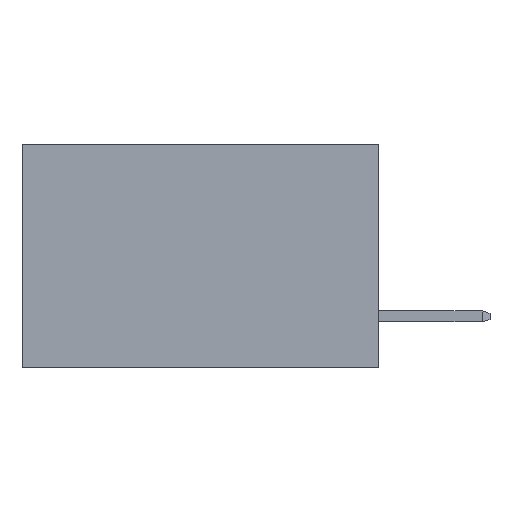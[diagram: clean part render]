
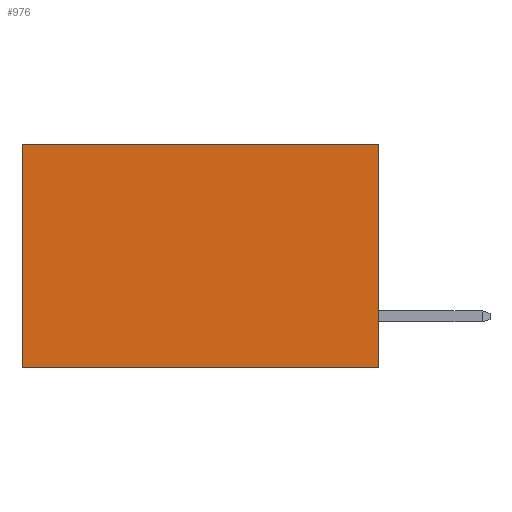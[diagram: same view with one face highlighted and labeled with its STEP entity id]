
A CAD part, left-side view. The second image highlights one B-rep face of the part: STEP entity #976.
In plain terms, the highlighted planar face has unit normal (-1, 0, 0).
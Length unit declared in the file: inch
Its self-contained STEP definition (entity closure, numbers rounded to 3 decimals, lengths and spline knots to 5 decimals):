
#169 = CARTESIAN_POINT ( 'NONE',  ( 0.277, 0., -0.37 ) ) ;
#976 = ADVANCED_FACE ( 'NONE', ( #1523 ), #10829, .F. ) ;
#1224 = DIRECTION ( 'NONE',  ( 0., 1., 0. ) ) ;
#1523 = FACE_OUTER_BOUND ( 'NONE', #5563, .T. ) ;
#1604 = EDGE_CURVE ( 'NONE', #8723, #1675, #9180, .T. ) ;
#1675 = VERTEX_POINT ( 'NONE', #10367 ) ;
#1906 = ORIENTED_EDGE ( 'NONE', *, *, #6919, .F. ) ;
#2808 = VECTOR ( 'NONE', #1224, 39.37008 ) ;
#2923 = EDGE_CURVE ( 'NONE', #1675, #7346, #4259, .T. ) ;
#3190 = CARTESIAN_POINT ( 'NONE',  ( 0.277, 0., 0. ) ) ;
#3775 = DIRECTION ( 'NONE',  ( 0., 0., -1. ) ) ;
#3964 = ORIENTED_EDGE ( 'NONE', *, *, #2923, .T. ) ;
#4161 = DIRECTION ( 'NONE',  ( 1., 0., 0. ) ) ;
#4244 = ORIENTED_EDGE ( 'NONE', *, *, #1604, .T. ) ;
#4259 = LINE ( 'NONE', #6363, #10473 ) ;
#5044 = LINE ( 'NONE', #10152, #6714 ) ;
#5308 = AXIS2_PLACEMENT_3D ( 'NONE', #169, #4161, #3775 ) ;
#5563 = EDGE_LOOP ( 'NONE', ( #3964, #6229, #1906, #4244 ) ) ;
#5669 = VERTEX_POINT ( 'NONE', #6389 ) ;
#6031 = CARTESIAN_POINT ( 'NONE',  ( 0.277, 0.59, -0.37 ) ) ;
#6229 = ORIENTED_EDGE ( 'NONE', *, *, #6674, .F. ) ;
#6363 = CARTESIAN_POINT ( 'NONE',  ( 0.277, 0.59, -0.37 ) ) ;
#6389 = CARTESIAN_POINT ( 'NONE',  ( 0.277, 0., -0.37 ) ) ;
#6674 = EDGE_CURVE ( 'NONE', #5669, #7346, #5044, .T. ) ;
#6714 = VECTOR ( 'NONE', #10219, 39.37008 ) ;
#6919 = EDGE_CURVE ( 'NONE', #8723, #5669, #6988, .T. ) ;
#6988 = LINE ( 'NONE', #8948, #10894 ) ;
#7187 = DIRECTION ( 'NONE',  ( 0., 0., -1. ) ) ;
#7346 = VERTEX_POINT ( 'NONE', #6031 ) ;
#8050 = CARTESIAN_POINT ( 'NONE',  ( 0.277, 0., 0. ) ) ;
#8723 = VERTEX_POINT ( 'NONE', #3190 ) ;
#8948 = CARTESIAN_POINT ( 'NONE',  ( 0.277, 0., -0.37 ) ) ;
#8969 = DIRECTION ( 'NONE',  ( 0., 0., -1. ) ) ;
#9180 = LINE ( 'NONE', #8050, #2808 ) ;
#10152 = CARTESIAN_POINT ( 'NONE',  ( 0.277, 0., -0.37 ) ) ;
#10219 = DIRECTION ( 'NONE',  ( 0., 1., 0. ) ) ;
#10367 = CARTESIAN_POINT ( 'NONE',  ( 0.277, 0.59, 0. ) ) ;
#10473 = VECTOR ( 'NONE', #7187, 39.37008 ) ;
#10829 = PLANE ( 'NONE',  #5308 ) ;
#10894 = VECTOR ( 'NONE', #8969, 39.37008 ) ;
